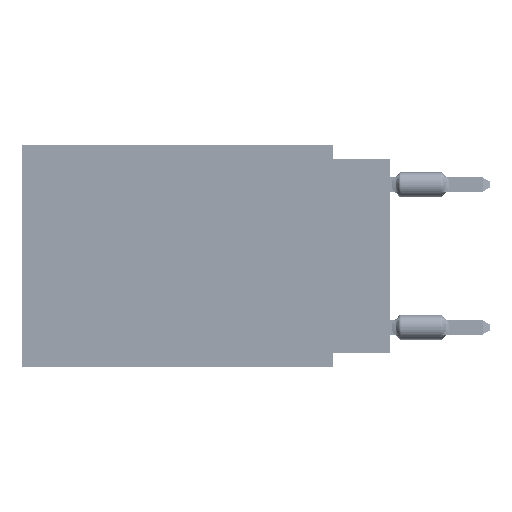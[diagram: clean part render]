
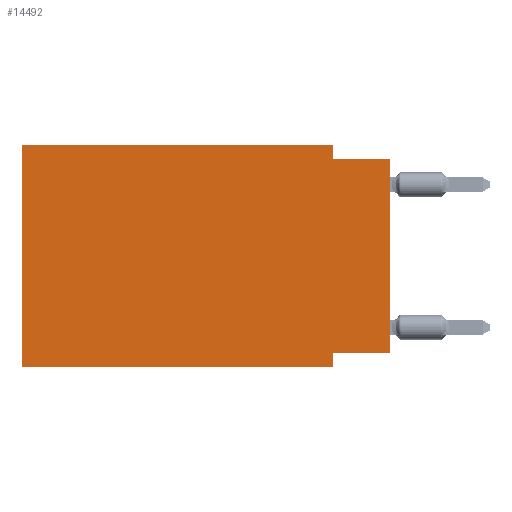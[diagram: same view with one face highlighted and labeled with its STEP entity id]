
A CAD part, left-side view. The second image highlights one B-rep face of the part: STEP entity #14492.
In plain terms, the highlighted planar face has unit normal (-1, 0, 0).
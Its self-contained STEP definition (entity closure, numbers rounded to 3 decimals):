
#237 = CARTESIAN_POINT ( 'NONE',  ( 0., 2.54, 0. ) ) ;
#3074 = CARTESIAN_POINT ( 'NONE',  ( 0., 16.383, 0. ) ) ;
#3400 = CARTESIAN_POINT ( 'NONE',  ( 0., 16.383, 0. ) ) ;
#5174 = DIRECTION ( 'NONE',  ( 0., 1., 0. ) ) ;
#7197 = EDGE_CURVE ( 'NONE', #25189, #22004, #8811, .T. ) ;
#8811 = LINE ( 'NONE', #57922, #25747 ) ;
#9177 = CARTESIAN_POINT ( 'NONE',  ( 0., 2.54, -0.635 ) ) ;
#10482 = EDGE_CURVE ( 'NONE', #36658, #28338, #56630, .T. ) ;
#12236 = EDGE_CURVE ( 'NONE', #29571, #43949, #13129, .T. ) ;
#13129 = LINE ( 'NONE', #50495, #21008 ) ;
#13532 = DIRECTION ( 'NONE',  ( 0., -1., 0. ) ) ;
#14492 = ADVANCED_FACE ( 'NONE', ( #39847 ), #33381, .F. ) ;
#14780 = ORIENTED_EDGE ( 'NONE', *, *, #12236, .F. ) ;
#15637 = LINE ( 'NONE', #3400, #39707 ) ;
#16357 = DIRECTION ( 'NONE',  ( 0., 0., 1. ) ) ;
#17765 = CARTESIAN_POINT ( 'NONE',  ( 0., 0., -9.271 ) ) ;
#18494 = DIRECTION ( 'NONE',  ( 0., 0., -1. ) ) ;
#18952 = LINE ( 'NONE', #237, #36664 ) ;
#19454 = VECTOR ( 'NONE', #18494, 1000. ) ;
#19885 = AXIS2_PLACEMENT_3D ( 'NONE', #70281, #25711, #76378 ) ;
#20804 = CARTESIAN_POINT ( 'NONE',  ( 0., 0., -0.635 ) ) ;
#21008 = VECTOR ( 'NONE', #13532, 1000. ) ;
#22004 = VERTEX_POINT ( 'NONE', #47065 ) ;
#22475 = VERTEX_POINT ( 'NONE', #35989 ) ;
#25189 = VERTEX_POINT ( 'NONE', #3074 ) ;
#25711 = DIRECTION ( 'NONE',  ( 1., 0., 0. ) ) ;
#25747 = VECTOR ( 'NONE', #26297, 1000. ) ;
#26297 = DIRECTION ( 'NONE',  ( 0., -1., 0. ) ) ;
#27712 = ORIENTED_EDGE ( 'NONE', *, *, #40890, .T. ) ;
#28338 = VERTEX_POINT ( 'NONE', #34793 ) ;
#29571 = VERTEX_POINT ( 'NONE', #9177 ) ;
#31791 = ORIENTED_EDGE ( 'NONE', *, *, #37477, .T. ) ;
#33381 = PLANE ( 'NONE',  #19885 ) ;
#34284 = DIRECTION ( 'NONE',  ( 0., 0., 1. ) ) ;
#34793 = CARTESIAN_POINT ( 'NONE',  ( 0., 2.54, -9.906 ) ) ;
#35989 = CARTESIAN_POINT ( 'NONE',  ( 0., 0., -9.271 ) ) ;
#36658 = VERTEX_POINT ( 'NONE', #40006 ) ;
#36664 = VECTOR ( 'NONE', #37630, 1000. ) ;
#37477 = EDGE_CURVE ( 'NONE', #45693, #28338, #40108, .T. ) ;
#37630 = DIRECTION ( 'NONE',  ( 0., 0., -1. ) ) ;
#38366 = CARTESIAN_POINT ( 'NONE',  ( 0., 2.54, -9.906 ) ) ;
#39707 = VECTOR ( 'NONE', #34284, 1000. ) ;
#39847 = FACE_OUTER_BOUND ( 'NONE', #77255, .T. ) ;
#40006 = CARTESIAN_POINT ( 'NONE',  ( 0., 2.54, -9.271 ) ) ;
#40108 = LINE ( 'NONE', #70931, #43492 ) ;
#40890 = EDGE_CURVE ( 'NONE', #22475, #43949, #47196, .T. ) ;
#41774 = EDGE_CURVE ( 'NONE', #22004, #29571, #18952, .T. ) ;
#42162 = VECTOR ( 'NONE', #5174, 1000. ) ;
#43492 = VECTOR ( 'NONE', #51518, 1000. ) ;
#43949 = VERTEX_POINT ( 'NONE', #20804 ) ;
#45693 = VERTEX_POINT ( 'NONE', #49520 ) ;
#47065 = CARTESIAN_POINT ( 'NONE',  ( 0., 2.54, 0. ) ) ;
#47196 = LINE ( 'NONE', #59368, #62491 ) ;
#47941 = EDGE_CURVE ( 'NONE', #45693, #25189, #15637, .T. ) ;
#49520 = CARTESIAN_POINT ( 'NONE',  ( 0., 16.383, -9.906 ) ) ;
#50495 = CARTESIAN_POINT ( 'NONE',  ( 0., 0., -0.635 ) ) ;
#51518 = DIRECTION ( 'NONE',  ( 0., -1., 0. ) ) ;
#53780 = ORIENTED_EDGE ( 'NONE', *, *, #58939, .F. ) ;
#54621 = ORIENTED_EDGE ( 'NONE', *, *, #7197, .F. ) ;
#56630 = LINE ( 'NONE', #38366, #19454 ) ;
#57922 = CARTESIAN_POINT ( 'NONE',  ( 0., 16.383, 0. ) ) ;
#58939 = EDGE_CURVE ( 'NONE', #22475, #36658, #66850, .T. ) ;
#59368 = CARTESIAN_POINT ( 'NONE',  ( 0., 0., 0. ) ) ;
#62491 = VECTOR ( 'NONE', #16357, 1000. ) ;
#66850 = LINE ( 'NONE', #17765, #42162 ) ;
#67876 = ORIENTED_EDGE ( 'NONE', *, *, #10482, .F. ) ;
#70207 = ORIENTED_EDGE ( 'NONE', *, *, #47941, .F. ) ;
#70281 = CARTESIAN_POINT ( 'NONE',  ( 0., 16.383, 0. ) ) ;
#70492 = ORIENTED_EDGE ( 'NONE', *, *, #41774, .F. ) ;
#70931 = CARTESIAN_POINT ( 'NONE',  ( 0., 16.383, -9.906 ) ) ;
#76378 = DIRECTION ( 'NONE',  ( 0., 0., -1. ) ) ;
#77255 = EDGE_LOOP ( 'NONE', ( #27712, #14780, #70492, #54621, #70207, #31791, #67876, #53780 ) ) ;
